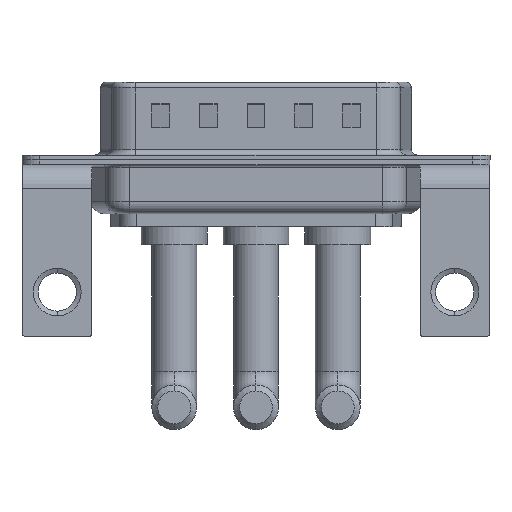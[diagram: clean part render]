
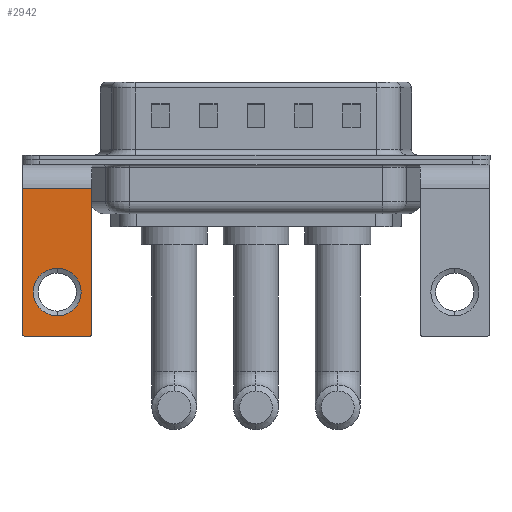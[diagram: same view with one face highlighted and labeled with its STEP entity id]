
A CAD part, front view. The second image highlights one B-rep face of the part: STEP entity #2942.
In plain terms, the highlighted planar face has unit normal (0, -1, 0).
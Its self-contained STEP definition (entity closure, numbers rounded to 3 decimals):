
#404 = CARTESIAN_POINT ( 'NONE',  ( 0., -6.25, -11.07 ) ) ;
#640 = DIRECTION ( 'NONE',  ( 0., 0., 1. ) ) ;
#835 = VERTEX_POINT ( 'NONE', #11988 ) ;
#1079 = CARTESIAN_POINT ( 'NONE',  ( 2.9, -6.25, -2.4 ) ) ;
#1169 = EDGE_CURVE ( 'NONE', #13911, #13517, #12224, .T. ) ;
#1190 = EDGE_CURVE ( 'NONE', #13517, #13911, #8220, .T. ) ;
#1265 = CARTESIAN_POINT ( 'NONE',  ( -2.65, -6.25, -14.55 ) ) ;
#1295 = EDGE_CURVE ( 'NONE', #4163, #14735, #14515, .T. ) ;
#1428 = VECTOR ( 'NONE', #3232, 1000. ) ;
#2000 = CARTESIAN_POINT ( 'NONE',  ( 2.9, -6.25, -14.8 ) ) ;
#2115 = ORIENTED_EDGE ( 'NONE', *, *, #9411, .F. ) ;
#2257 = CARTESIAN_POINT ( 'NONE',  ( -2.9, -6.25, -2.4 ) ) ;
#2301 = ORIENTED_EDGE ( 'NONE', *, *, #1295, .T. ) ;
#2477 = ORIENTED_EDGE ( 'NONE', *, *, #15987, .T. ) ;
#2523 = EDGE_LOOP ( 'NONE', ( #11059, #14246 ) ) ;
#2801 = EDGE_CURVE ( 'NONE', #11787, #5875, #5900, .T. ) ;
#2882 = CARTESIAN_POINT ( 'NONE',  ( 0., -6.25, -11.07 ) ) ;
#2942 = ADVANCED_FACE ( 'NONE', ( #7374, #12463 ), #10873, .F. ) ;
#2966 = DIRECTION ( 'NONE',  ( 0., 1., 0. ) ) ;
#3232 = DIRECTION ( 'NONE',  ( 0., 0., -1. ) ) ;
#3250 = DIRECTION ( 'NONE',  ( -1., 0., 0. ) ) ;
#3888 = DIRECTION ( 'NONE',  ( 0., 1., 0. ) ) ;
#4163 = VERTEX_POINT ( 'NONE', #9385 ) ;
#4778 = CIRCLE ( 'NONE', #13527, 0.25 ) ;
#5709 = CARTESIAN_POINT ( 'NONE',  ( 2.9, -6.25, -2.4 ) ) ;
#5744 = VECTOR ( 'NONE', #3250, 1000. ) ;
#5875 = VERTEX_POINT ( 'NONE', #16170 ) ;
#5898 = DIRECTION ( 'NONE',  ( 0., 1., 0. ) ) ;
#5900 = CIRCLE ( 'NONE', #8023, 0.25 ) ;
#5988 = DIRECTION ( 'NONE',  ( 0., 0., 1. ) ) ;
#6539 = ORIENTED_EDGE ( 'NONE', *, *, #11924, .T. ) ;
#6699 = CARTESIAN_POINT ( 'NONE',  ( 2.65, -6.25, -14.8 ) ) ;
#6899 = AXIS2_PLACEMENT_3D ( 'NONE', #2882, #3888, #9194 ) ;
#6996 = DIRECTION ( 'NONE',  ( 0., 0., -1. ) ) ;
#7374 = FACE_BOUND ( 'NONE', #2523, .T. ) ;
#7897 = DIRECTION ( 'NONE',  ( 0., 0., 1. ) ) ;
#8023 = AXIS2_PLACEMENT_3D ( 'NONE', #11738, #14621, #7897 ) ;
#8220 = CIRCLE ( 'NONE', #12486, 2. ) ;
#9030 = CARTESIAN_POINT ( 'NONE',  ( 0., -6.25, -9.07 ) ) ;
#9068 = CARTESIAN_POINT ( 'NONE',  ( -2.9, -6.25, -14.55 ) ) ;
#9194 = DIRECTION ( 'NONE',  ( 0., 0., 1. ) ) ;
#9385 = CARTESIAN_POINT ( 'NONE',  ( 2.9, -6.25, -2.4 ) ) ;
#9411 = EDGE_CURVE ( 'NONE', #11787, #835, #11905, .T. ) ;
#10158 = DIRECTION ( 'NONE',  ( 0., -1., 0. ) ) ;
#10640 = EDGE_LOOP ( 'NONE', ( #2477, #6539, #2115, #10871, #12651, #2301 ) ) ;
#10695 = DIRECTION ( 'NONE',  ( -1., 0., 0. ) ) ;
#10865 = LINE ( 'NONE', #10959, #1428 ) ;
#10871 = ORIENTED_EDGE ( 'NONE', *, *, #2801, .T. ) ;
#10873 = PLANE ( 'NONE',  #13337 ) ;
#10959 = CARTESIAN_POINT ( 'NONE',  ( -2.9, -6.25, -2.4 ) ) ;
#11059 = ORIENTED_EDGE ( 'NONE', *, *, #1169, .T. ) ;
#11623 = EDGE_CURVE ( 'NONE', #4163, #5875, #12081, .T. ) ;
#11738 = CARTESIAN_POINT ( 'NONE',  ( 2.65, -6.25, -14.55 ) ) ;
#11787 = VERTEX_POINT ( 'NONE', #6699 ) ;
#11905 = LINE ( 'NONE', #2000, #5744 ) ;
#11924 = EDGE_CURVE ( 'NONE', #13005, #835, #4778, .T. ) ;
#11988 = CARTESIAN_POINT ( 'NONE',  ( -2.65, -6.25, -14.8 ) ) ;
#12081 = LINE ( 'NONE', #15893, #14062 ) ;
#12224 = CIRCLE ( 'NONE', #6899, 2. ) ;
#12463 = FACE_OUTER_BOUND ( 'NONE', #10640, .T. ) ;
#12486 = AXIS2_PLACEMENT_3D ( 'NONE', #404, #2966, #640 ) ;
#12651 = ORIENTED_EDGE ( 'NONE', *, *, #11623, .F. ) ;
#13005 = VERTEX_POINT ( 'NONE', #9068 ) ;
#13337 = AXIS2_PLACEMENT_3D ( 'NONE', #1079, #5898, #5988 ) ;
#13517 = VERTEX_POINT ( 'NONE', #9030 ) ;
#13527 = AXIS2_PLACEMENT_3D ( 'NONE', #1265, #10158, #14989 ) ;
#13911 = VERTEX_POINT ( 'NONE', #16265 ) ;
#14062 = VECTOR ( 'NONE', #6996, 1000. ) ;
#14246 = ORIENTED_EDGE ( 'NONE', *, *, #1190, .T. ) ;
#14344 = VECTOR ( 'NONE', #10695, 1000. ) ;
#14515 = LINE ( 'NONE', #5709, #14344 ) ;
#14621 = DIRECTION ( 'NONE',  ( 0., -1., 0. ) ) ;
#14735 = VERTEX_POINT ( 'NONE', #2257 ) ;
#14989 = DIRECTION ( 'NONE',  ( 0., 0., 1. ) ) ;
#15893 = CARTESIAN_POINT ( 'NONE',  ( 2.9, -6.25, -2.4 ) ) ;
#15987 = EDGE_CURVE ( 'NONE', #14735, #13005, #10865, .T. ) ;
#16170 = CARTESIAN_POINT ( 'NONE',  ( 2.9, -6.25, -14.55 ) ) ;
#16265 = CARTESIAN_POINT ( 'NONE',  ( 0., -6.25, -13.07 ) ) ;
